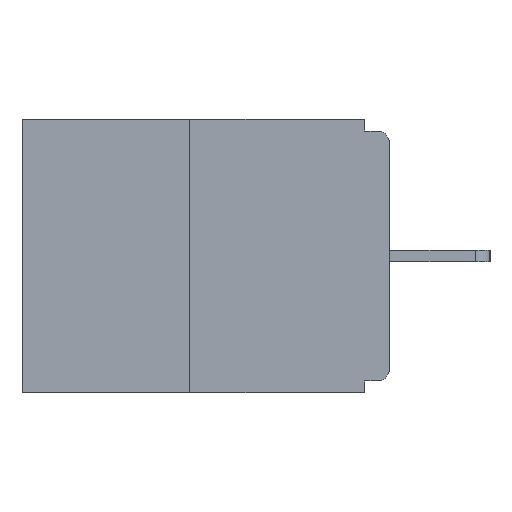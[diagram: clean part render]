
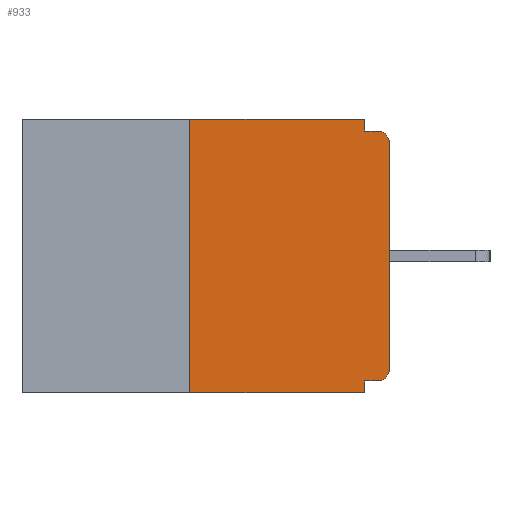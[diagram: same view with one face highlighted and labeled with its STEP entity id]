
A CAD part, left-side view. The second image highlights one B-rep face of the part: STEP entity #933.
In plain terms, the highlighted planar face has unit normal (-1, 0, 0).
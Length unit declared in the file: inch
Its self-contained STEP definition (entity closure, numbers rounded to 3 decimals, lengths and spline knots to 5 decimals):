
#86 = VECTOR ( 'NONE', #14911, 39.37008 ) ;
#150 = ORIENTED_EDGE ( 'NONE', *, *, #11708, .F. ) ;
#436 = EDGE_CURVE ( 'NONE', #3312, #5550, #12836, .T. ) ;
#445 = VECTOR ( 'NONE', #22683, 39.37008 ) ;
#675 = AXIS2_PLACEMENT_3D ( 'NONE', #5390, #1972, #1948 ) ;
#933 = ADVANCED_FACE ( 'NONE', ( #18068 ), #23051, .F. ) ;
#991 = VECTOR ( 'NONE', #12049, 39.37008 ) ;
#1424 = ORIENTED_EDGE ( 'NONE', *, *, #16233, .F. ) ;
#1948 = DIRECTION ( 'NONE',  ( 0., 0., -1. ) ) ;
#1972 = DIRECTION ( 'NONE',  ( -1., 0., 0. ) ) ;
#2040 = LINE ( 'NONE', #11186, #11922 ) ;
#2640 = ORIENTED_EDGE ( 'NONE', *, *, #3064, .T. ) ;
#3064 = EDGE_CURVE ( 'NONE', #6301, #12479, #17604, .T. ) ;
#3243 = ORIENTED_EDGE ( 'NONE', *, *, #15361, .T. ) ;
#3312 = VERTEX_POINT ( 'NONE', #3680 ) ;
#3680 = CARTESIAN_POINT ( 'NONE',  ( 0., 0., -0.03 ) ) ;
#5218 = LINE ( 'NONE', #21812, #86 ) ;
#5310 = VECTOR ( 'NONE', #15478, 39.37008 ) ;
#5390 = CARTESIAN_POINT ( 'NONE',  ( 0., 0.015, -0.313 ) ) ;
#5438 = VERTEX_POINT ( 'NONE', #19666 ) ;
#5550 = VERTEX_POINT ( 'NONE', #13831 ) ;
#5581 = EDGE_CURVE ( 'NONE', #17243, #5550, #12464, .T. ) ;
#6075 = CARTESIAN_POINT ( 'NONE',  ( 0., 0.25, -0.343 ) ) ;
#6301 = VERTEX_POINT ( 'NONE', #8199 ) ;
#7288 = EDGE_LOOP ( 'NONE', ( #150, #14998, #20166, #1424, #11907, #2640, #3243, #8198, #13609, #18320 ) ) ;
#8189 = CARTESIAN_POINT ( 'NONE',  ( 0., 0., 0. ) ) ;
#8198 = ORIENTED_EDGE ( 'NONE', *, *, #436, .T. ) ;
#8199 = CARTESIAN_POINT ( 'NONE',  ( 0., 0.015, -0.328 ) ) ;
#8544 = VERTEX_POINT ( 'NONE', #10614 ) ;
#9624 = VERTEX_POINT ( 'NONE', #15884 ) ;
#10543 = EDGE_CURVE ( 'NONE', #6301, #8544, #5218, .T. ) ;
#10614 = CARTESIAN_POINT ( 'NONE',  ( 0., 0.031, -0.328 ) ) ;
#10875 = AXIS2_PLACEMENT_3D ( 'NONE', #12233, #11503, #11239 ) ;
#11186 = CARTESIAN_POINT ( 'NONE',  ( 0., 0.031, 0. ) ) ;
#11239 = DIRECTION ( 'NONE',  ( 0., 0., -1. ) ) ;
#11503 = DIRECTION ( 'NONE',  ( -1., 0., 0. ) ) ;
#11708 = EDGE_CURVE ( 'NONE', #5438, #15250, #15722, .T. ) ;
#11860 = DIRECTION ( 'NONE',  ( 0., 0., 1. ) ) ;
#11907 = ORIENTED_EDGE ( 'NONE', *, *, #10543, .F. ) ;
#11922 = VECTOR ( 'NONE', #21682, 39.37008 ) ;
#12019 = LINE ( 'NONE', #8189, #13161 ) ;
#12049 = DIRECTION ( 'NONE',  ( 0., -1., 0. ) ) ;
#12233 = CARTESIAN_POINT ( 'NONE',  ( 0., 0.015, -0.03 ) ) ;
#12298 = CARTESIAN_POINT ( 'NONE',  ( 0., 0.25, 0. ) ) ;
#12464 = LINE ( 'NONE', #13217, #21748 ) ;
#12479 = VERTEX_POINT ( 'NONE', #22649 ) ;
#12836 = CIRCLE ( 'NONE', #10875, 0.015 ) ;
#13161 = VECTOR ( 'NONE', #11860, 39.37008 ) ;
#13217 = CARTESIAN_POINT ( 'NONE',  ( 0., 0., -0.015 ) ) ;
#13295 = DIRECTION ( 'NONE',  ( 0., -1., 0. ) ) ;
#13609 = ORIENTED_EDGE ( 'NONE', *, *, #5581, .F. ) ;
#13831 = CARTESIAN_POINT ( 'NONE',  ( 0., 0.015, -0.015 ) ) ;
#14911 = DIRECTION ( 'NONE',  ( 0., 1., 0. ) ) ;
#14998 = ORIENTED_EDGE ( 'NONE', *, *, #18590, .F. ) ;
#15048 = EDGE_CURVE ( 'NONE', #15250, #17243, #2040, .T. ) ;
#15244 = LINE ( 'NONE', #12298, #445 ) ;
#15250 = VERTEX_POINT ( 'NONE', #22067 ) ;
#15361 = EDGE_CURVE ( 'NONE', #12479, #3312, #12019, .T. ) ;
#15478 = DIRECTION ( 'NONE',  ( 0., -1., 0. ) ) ;
#15591 = CARTESIAN_POINT ( 'NONE',  ( 0., 0.46, 0. ) ) ;
#15722 = LINE ( 'NONE', #15591, #991 ) ;
#15751 = CARTESIAN_POINT ( 'NONE',  ( 0., 0.031, -0.343 ) ) ;
#15884 = CARTESIAN_POINT ( 'NONE',  ( 0., 0.031, -0.343 ) ) ;
#16233 = EDGE_CURVE ( 'NONE', #8544, #9624, #22932, .T. ) ;
#16496 = DIRECTION ( 'NONE',  ( 0., 0., -1. ) ) ;
#17243 = VERTEX_POINT ( 'NONE', #18557 ) ;
#17409 = EDGE_CURVE ( 'NONE', #22102, #9624, #17792, .T. ) ;
#17604 = CIRCLE ( 'NONE', #675, 0.015 ) ;
#17792 = LINE ( 'NONE', #20612, #5310 ) ;
#18068 = FACE_OUTER_BOUND ( 'NONE', #7288, .T. ) ;
#18320 = ORIENTED_EDGE ( 'NONE', *, *, #15048, .F. ) ;
#18385 = VECTOR ( 'NONE', #22697, 39.37008 ) ;
#18557 = CARTESIAN_POINT ( 'NONE',  ( 0., 0.031, -0.015 ) ) ;
#18590 = EDGE_CURVE ( 'NONE', #22102, #5438, #15244, .T. ) ;
#19666 = CARTESIAN_POINT ( 'NONE',  ( 0., 0.25, 0. ) ) ;
#20166 = ORIENTED_EDGE ( 'NONE', *, *, #17409, .T. ) ;
#20612 = CARTESIAN_POINT ( 'NONE',  ( 0., 0.46, -0.343 ) ) ;
#20810 = CARTESIAN_POINT ( 'NONE',  ( 0., 0.46, 0. ) ) ;
#20858 = DIRECTION ( 'NONE',  ( 1., 0., 0. ) ) ;
#21682 = DIRECTION ( 'NONE',  ( 0., 0., -1. ) ) ;
#21748 = VECTOR ( 'NONE', #13295, 39.37008 ) ;
#21753 = AXIS2_PLACEMENT_3D ( 'NONE', #20810, #20858, #16496 ) ;
#21812 = CARTESIAN_POINT ( 'NONE',  ( 0., 0., -0.328 ) ) ;
#22067 = CARTESIAN_POINT ( 'NONE',  ( 0., 0.031, 0. ) ) ;
#22102 = VERTEX_POINT ( 'NONE', #6075 ) ;
#22649 = CARTESIAN_POINT ( 'NONE',  ( 0., 0., -0.313 ) ) ;
#22683 = DIRECTION ( 'NONE',  ( 0., 0., 1. ) ) ;
#22697 = DIRECTION ( 'NONE',  ( 0., 0., -1. ) ) ;
#22932 = LINE ( 'NONE', #15751, #18385 ) ;
#23051 = PLANE ( 'NONE',  #21753 ) ;
